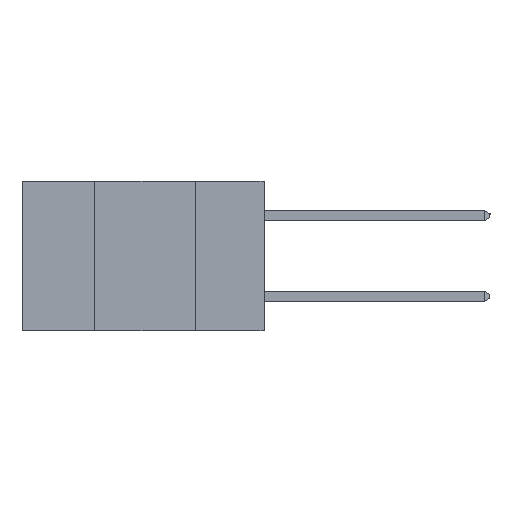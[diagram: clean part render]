
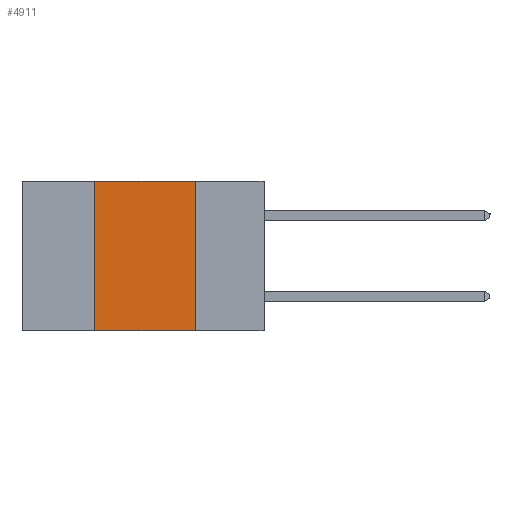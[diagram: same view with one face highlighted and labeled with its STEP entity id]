
A CAD part, left-side view. The second image highlights one B-rep face of the part: STEP entity #4911.
In plain terms, the highlighted planar face has unit normal (-1, 0, 0).
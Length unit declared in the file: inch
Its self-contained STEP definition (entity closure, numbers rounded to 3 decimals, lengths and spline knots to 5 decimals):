
#891 = EDGE_LOOP ( 'NONE', ( #7540, #13975, #11962, #2584 ) ) ;
#1607 = DIRECTION ( 'NONE',  ( 0., 0., -1. ) ) ;
#2142 = CARTESIAN_POINT ( 'NONE',  ( 0., 0.17, 0. ) ) ;
#2258 = CARTESIAN_POINT ( 'NONE',  ( 0., 0.42, -0.37 ) ) ;
#2557 = VERTEX_POINT ( 'NONE', #6974 ) ;
#2584 = ORIENTED_EDGE ( 'NONE', *, *, #3883, .T. ) ;
#3280 = DIRECTION ( 'NONE',  ( 0., 0., 1. ) ) ;
#3372 = CARTESIAN_POINT ( 'NONE',  ( 0., 0.6, 0. ) ) ;
#3442 = AXIS2_PLACEMENT_3D ( 'NONE', #10897, #12232, #1607 ) ;
#3528 = LINE ( 'NONE', #4551, #8623 ) ;
#3883 = EDGE_CURVE ( 'NONE', #10531, #2557, #3528, .T. ) ;
#4475 = LINE ( 'NONE', #3372, #7636 ) ;
#4551 = CARTESIAN_POINT ( 'NONE',  ( 0., 0.6, -0.37 ) ) ;
#4911 = ADVANCED_FACE ( 'NONE', ( #9831 ), #7532, .F. ) ;
#5084 = LINE ( 'NONE', #9806, #7413 ) ;
#5733 = DIRECTION ( 'NONE',  ( 0., -1., 0. ) ) ;
#6164 = VERTEX_POINT ( 'NONE', #2142 ) ;
#6263 = VERTEX_POINT ( 'NONE', #9756 ) ;
#6974 = CARTESIAN_POINT ( 'NONE',  ( 0., 0.17, -0.37 ) ) ;
#7413 = VECTOR ( 'NONE', #13389, 39.37008 ) ;
#7532 = PLANE ( 'NONE',  #3442 ) ;
#7540 = ORIENTED_EDGE ( 'NONE', *, *, #13350, .F. ) ;
#7636 = VECTOR ( 'NONE', #12986, 39.37008 ) ;
#8623 = VECTOR ( 'NONE', #5733, 39.37008 ) ;
#9756 = CARTESIAN_POINT ( 'NONE',  ( 0., 0.42, 0. ) ) ;
#9806 = CARTESIAN_POINT ( 'NONE',  ( 0., 0.17, -0.37 ) ) ;
#9815 = EDGE_CURVE ( 'NONE', #6263, #6164, #4475, .T. ) ;
#9831 = FACE_OUTER_BOUND ( 'NONE', #891, .T. ) ;
#10531 = VERTEX_POINT ( 'NONE', #12267 ) ;
#10897 = CARTESIAN_POINT ( 'NONE',  ( 0., 0.6, 0. ) ) ;
#11502 = EDGE_CURVE ( 'NONE', #10531, #6263, #12903, .T. ) ;
#11962 = ORIENTED_EDGE ( 'NONE', *, *, #11502, .F. ) ;
#12232 = DIRECTION ( 'NONE',  ( 1., 0., 0. ) ) ;
#12267 = CARTESIAN_POINT ( 'NONE',  ( 0., 0.42, -0.37 ) ) ;
#12590 = VECTOR ( 'NONE', #3280, 39.37008 ) ;
#12903 = LINE ( 'NONE', #2258, #12590 ) ;
#12986 = DIRECTION ( 'NONE',  ( 0., -1., 0. ) ) ;
#13350 = EDGE_CURVE ( 'NONE', #6164, #2557, #5084, .T. ) ;
#13389 = DIRECTION ( 'NONE',  ( 0., 0., -1. ) ) ;
#13975 = ORIENTED_EDGE ( 'NONE', *, *, #9815, .F. ) ;
